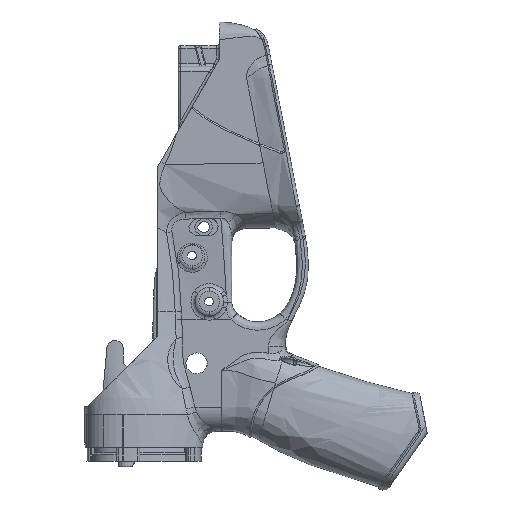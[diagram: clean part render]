
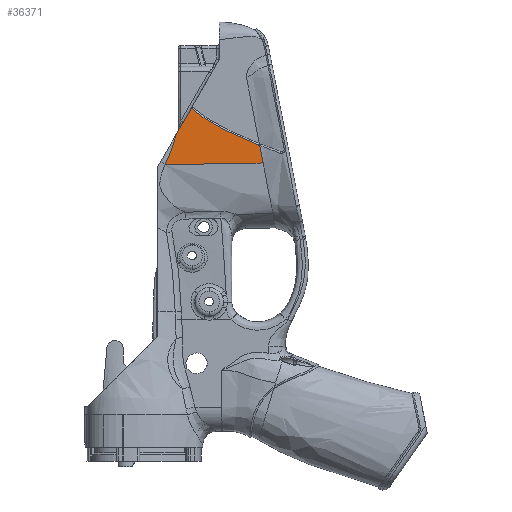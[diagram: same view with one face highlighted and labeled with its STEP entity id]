
A CAD part, left-side view. The second image highlights one B-rep face of the part: STEP entity #36371.
In plain terms, the highlighted planar face has unit normal (-1, 0, 0).
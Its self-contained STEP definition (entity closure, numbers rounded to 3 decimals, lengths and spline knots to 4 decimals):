
#1623 = CARTESIAN_POINT ( 'NONE',  ( -0.7, -2.4807, -1.2377 ) ) ;
#3707 = CARTESIAN_POINT ( 'NONE',  ( -0.7, -1.4744, -0.7435 ) ) ;
#3806 = DIRECTION ( 'NONE',  ( 0., -0.191, -0.982 ) ) ;
#4633 = LINE ( 'NONE', #80632, #74963 ) ;
#5125 = ORIENTED_EDGE ( 'NONE', *, *, #51170, .T. ) ;
#7297 = LINE ( 'NONE', #40493, #68315 ) ;
#7760 = VERTEX_POINT ( 'NONE', #69043 ) ;
#11042 = CARTESIAN_POINT ( 'NONE',  ( -0.7, -2.5482, -1.5611 ) ) ;
#11452 = CARTESIAN_POINT ( 'NONE',  ( -0.7, -0.9198, -1.2056 ) ) ;
#11867 = CARTESIAN_POINT ( 'NONE',  ( -0.7, -0.882, -1.3142 ) ) ;
#13428 = CARTESIAN_POINT ( 'NONE',  ( -0.7, -2.4857, -1.2395 ) ) ;
#14308 = VECTOR ( 'NONE', #60635, 39.3701 ) ;
#16718 = CARTESIAN_POINT ( 'NONE',  ( -0.7, -2.0393, -1.0514 ) ) ;
#17656 = B_SPLINE_CURVE_WITH_KNOTS ( 'NONE', 3,
 ( #67940, #54932, #56154, #16718, #81358, #49074, #42782, #23021, #36070, #61637, #3707, #30150, #80948, #22607, #81768, #23425 ),
 .UNSPECIFIED., .F., .F.,
 ( 4, 2, 2, 2, 2, 2, 2, 4 ),
 ( 0., 0.0089, 0.0178, 0.0223, 0.0267, 0.029, 0.0312, 0.0356 ),
 .UNSPECIFIED. ) ;
#18575 = CARTESIAN_POINT ( 'NONE',  ( -0.7, -0.9512, -1.0955 ) ) ;
#19054 = EDGE_CURVE ( 'NONE', #46935, #41538, #52037, .T. ) ;
#20103 = CARTESIAN_POINT ( 'NONE',  ( -0.7, -2.4758, -1.2359 ) ) ;
#22607 = CARTESIAN_POINT ( 'NONE',  ( -0.7, -1.3309, -0.6396 ) ) ;
#22850 = DIRECTION ( 'NONE',  ( 0., 0., 1. ) ) ;
#23021 = CARTESIAN_POINT ( 'NONE',  ( -0.7, -1.6236, -0.8371 ) ) ;
#23425 = CARTESIAN_POINT ( 'NONE',  ( -0.7, -1.2426, -0.5623 ) ) ;
#24171 = CARTESIAN_POINT ( 'NONE',  ( -0.7, -0.7628, -1.5923 ) ) ;
#24841 = CARTESIAN_POINT ( 'NONE',  ( -0.7, -0.8479, -1.3982 ) ) ;
#25256 = CARTESIAN_POINT ( 'NONE',  ( -0.7, -0.8426, -1.4107 ) ) ;
#30150 = CARTESIAN_POINT ( 'NONE',  ( -0.7, -1.4258, -0.71 ) ) ;
#33551 = CARTESIAN_POINT ( 'NONE',  ( -0.7, -2.4832, -1.2386 ) ) ;
#33763 = DIRECTION ( 'NONE',  ( 0., 0.5, -0.866 ) ) ;
#35469 = LINE ( 'NONE', #53929, #14308 ) ;
#36070 = CARTESIAN_POINT ( 'NONE',  ( -0.7, -1.5732, -0.8072 ) ) ;
#36313 = FACE_OUTER_BOUND ( 'NONE', #65394, .T. ) ;
#36371 = ADVANCED_FACE ( 'NONE', ( #36313 ), #56001, .T. ) ;
#36577 = ORIENTED_EDGE ( 'NONE', *, *, #60880, .T. ) ;
#37090 = CARTESIAN_POINT ( 'NONE',  ( -0.7, -0.8445, -1.4061 ) ) ;
#37501 = CARTESIAN_POINT ( 'NONE',  ( -0.7, -0.8611, -1.3666 ) ) ;
#37911 = CARTESIAN_POINT ( 'NONE',  ( -0.7, -0.7628, -1.5923 ) ) ;
#38318 = CARTESIAN_POINT ( 'NONE',  ( -0.7, -0.8247, -1.452 ) ) ;
#38573 = EDGE_CURVE ( 'NONE', #74006, #39544, #61642, .T. ) ;
#39442 = CARTESIAN_POINT ( 'NONE',  ( -0.7, -2.4709, -1.2341 ) ) ;
#39544 = VERTEX_POINT ( 'NONE', #43706 ) ;
#40493 = CARTESIAN_POINT ( 'NONE',  ( -0.7, -2.6175, 1.8191 ) ) ;
#41538 = VERTEX_POINT ( 'NONE', #24171 ) ;
#42059 = EDGE_CURVE ( 'NONE', #61138, #41538, #35469, .T. ) ;
#42782 = CARTESIAN_POINT ( 'NONE',  ( -0.7, -1.7255, -0.8946 ) ) ;
#43706 = CARTESIAN_POINT ( 'NONE',  ( -0.7, -2.4709, -1.2341 ) ) ;
#43793 = CARTESIAN_POINT ( 'NONE',  ( -0.7, -0.9367, -1.1517 ) ) ;
#44206 = CARTESIAN_POINT ( 'NONE',  ( -0.7, -0.8434, -1.4088 ) ) ;
#44607 = CARTESIAN_POINT ( 'NONE',  ( -0.7, -0.8982, -1.2699 ) ) ;
#46935 = VERTEX_POINT ( 'NONE', #50745 ) ;
#49074 = CARTESIAN_POINT ( 'NONE',  ( -0.7, -1.7771, -0.9221 ) ) ;
#49329 = CARTESIAN_POINT ( 'NONE',  ( -0.7, -3.8791, 1.0907 ) ) ;
#50745 = CARTESIAN_POINT ( 'NONE',  ( -0.7, -0.9615, -1.0491 ) ) ;
#51170 = EDGE_CURVE ( 'NONE', #39544, #7760, #17656, .T. ) ;
#52037 = B_SPLINE_CURVE_WITH_KNOTS ( 'NONE', 3,
 ( #75672, #18575, #43793, #11452, #69386, #82366, #44607, #11867, #37501, #24841, #37090, #57175, #76085, #44206, #70192, #25256, #69790, #38318, #63892, #37911 ),
 .UNSPECIFIED., .F., .F.,
 ( 4, 1, 2, 2, 1, 1, 1, 1, 2, 2, 1, 1, 1, 4 ),
 ( 0.6252, 0.7189, 0.7423, 0.7658, 0.8126, 0.8595, 0.8712, 0.8741, 0.8748, 0.8756, 0.877, 0.8829, 0.9063, 1. ),
 .UNSPECIFIED. ) ;
#53617 = ORIENTED_EDGE ( 'NONE', *, *, #19054, .T. ) ;
#53929 = CARTESIAN_POINT ( 'NONE',  ( -0.7, -3.925, -1.5371 ) ) ;
#54932 = CARTESIAN_POINT ( 'NONE',  ( -0.7, -2.3618, -1.1907 ) ) ;
#56001 = PLANE ( 'NONE',  #58369 ) ;
#56154 = CARTESIAN_POINT ( 'NONE',  ( -0.7, -2.2535, -1.1459 ) ) ;
#57175 = CARTESIAN_POINT ( 'NONE',  ( -0.7, -0.8437, -1.408 ) ) ;
#58369 = AXIS2_PLACEMENT_3D ( 'NONE', #49329, #81606, #22850 ) ;
#59141 = CARTESIAN_POINT ( 'NONE',  ( -0.7, -2.4857, -1.2395 ) ) ;
#60635 = DIRECTION ( 'NONE',  ( 0., 1., -0.017 ) ) ;
#60880 = EDGE_CURVE ( 'NONE', #7760, #46935, #7297, .T. ) ;
#61138 = VERTEX_POINT ( 'NONE', #11042 ) ;
#61251 = ORIENTED_EDGE ( 'NONE', *, *, #38573, .T. ) ;
#61637 = CARTESIAN_POINT ( 'NONE',  ( -0.7, -1.499, -0.7597 ) ) ;
#61642 = B_SPLINE_CURVE_WITH_KNOTS ( 'NONE', 3,
 ( #59141, #33551, #1623, #20103, #70911, #39442 ),
 .UNSPECIFIED., .F., .F.,
 ( 4, 2, 4 ),
 ( 0., 0.0002, 0.0004 ),
 .UNSPECIFIED. ) ;
#63892 = CARTESIAN_POINT ( 'NONE',  ( -0.7, -0.7956, -1.5182 ) ) ;
#65055 = EDGE_CURVE ( 'NONE', #74006, #61138, #4633, .T. ) ;
#65394 = EDGE_LOOP ( 'NONE', ( #5125, #36577, #53617, #67194, #70522, #61251 ) ) ;
#67194 = ORIENTED_EDGE ( 'NONE', *, *, #42059, .F. ) ;
#67940 = CARTESIAN_POINT ( 'NONE',  ( -0.7, -2.4709, -1.2341 ) ) ;
#68315 = VECTOR ( 'NONE', #33763, 39.3701 ) ;
#69043 = CARTESIAN_POINT ( 'NONE',  ( -0.7, -1.2426, -0.5623 ) ) ;
#69386 = CARTESIAN_POINT ( 'NONE',  ( -0.7, -0.9129, -1.227 ) ) ;
#69790 = CARTESIAN_POINT ( 'NONE',  ( -0.7, -0.8398, -1.4172 ) ) ;
#70192 = CARTESIAN_POINT ( 'NONE',  ( -0.7, -0.8432, -1.4092 ) ) ;
#70522 = ORIENTED_EDGE ( 'NONE', *, *, #65055, .F. ) ;
#70911 = CARTESIAN_POINT ( 'NONE',  ( -0.7, -2.4733, -1.235 ) ) ;
#74006 = VERTEX_POINT ( 'NONE', #13428 ) ;
#74963 = VECTOR ( 'NONE', #3806, 39.3701 ) ;
#75672 = CARTESIAN_POINT ( 'NONE',  ( -0.7, -0.9615, -1.0491 ) ) ;
#76085 = CARTESIAN_POINT ( 'NONE',  ( -0.7, -0.8434, -1.4088 ) ) ;
#80632 = CARTESIAN_POINT ( 'NONE',  ( -0.7, -2.2431, 0.0085 ) ) ;
#80948 = CARTESIAN_POINT ( 'NONE',  ( -0.7, -1.4017, -0.6928 ) ) ;
#81358 = CARTESIAN_POINT ( 'NONE',  ( -0.7, -1.9333, -1.0019 ) ) ;
#81606 = DIRECTION ( 'NONE',  ( -1., 0., 0. ) ) ;
#81768 = CARTESIAN_POINT ( 'NONE',  ( -0.7, -1.2855, -0.6023 ) ) ;
#82366 = CARTESIAN_POINT ( 'NONE',  ( -0.7, -0.9093, -1.2375 ) ) ;
